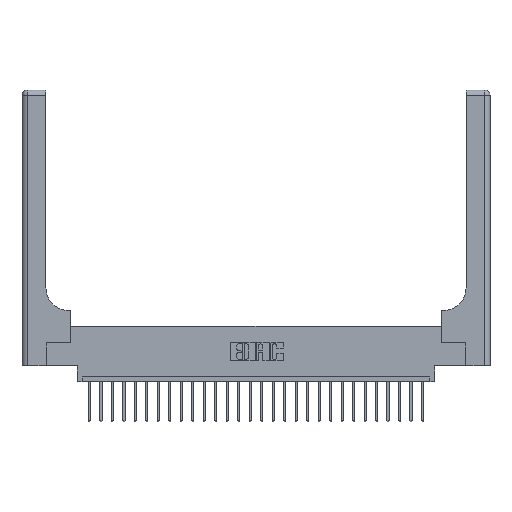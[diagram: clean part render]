
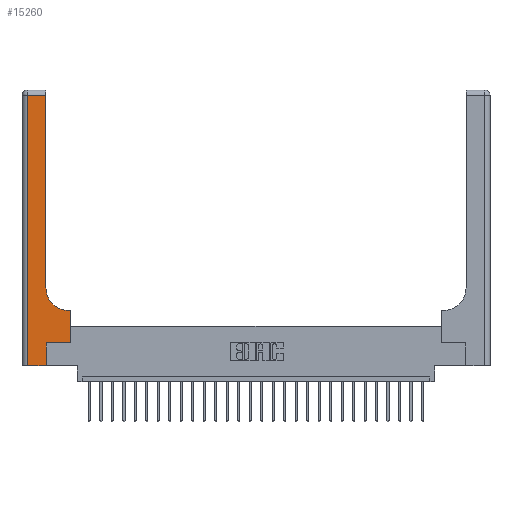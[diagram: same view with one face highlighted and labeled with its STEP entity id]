
A CAD part, top view. The second image highlights one B-rep face of the part: STEP entity #15260.
In plain terms, the highlighted planar face has unit normal (0, 0, 1).
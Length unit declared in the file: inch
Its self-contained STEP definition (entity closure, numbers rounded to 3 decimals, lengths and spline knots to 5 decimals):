
#6 = VERTEX_POINT ( 'NONE', #24282 ) ;
#152 = VECTOR ( 'NONE', #21282, 39.37008 ) ;
#178 = VECTOR ( 'NONE', #401, 39.37008 ) ;
#401 = DIRECTION ( 'NONE',  ( 0., 1., 0. ) ) ;
#1646 = EDGE_CURVE ( 'NONE', #12417, #21705, #16898, .T. ) ;
#3020 = VERTEX_POINT ( 'NONE', #6856 ) ;
#3327 = VECTOR ( 'NONE', #15377, 39.37008 ) ;
#3808 = EDGE_CURVE ( 'NONE', #14469, #10279, #16471, .T. ) ;
#3877 = ORIENTED_EDGE ( 'NONE', *, *, #6698, .T. ) ;
#3986 = EDGE_LOOP ( 'NONE', ( #5936, #6152, #3877, #6165, #24471, #15004, #22845, #21467, #20799 ) ) ;
#4319 = PLANE ( 'NONE',  #25416 ) ;
#4396 = CARTESIAN_POINT ( 'NONE',  ( 0.51, 0.6, 0.37 ) ) ;
#4500 = VERTEX_POINT ( 'NONE', #19045 ) ;
#4803 = CARTESIAN_POINT ( 'NONE',  ( 0., 0., 0.37 ) ) ;
#5450 = EDGE_CURVE ( 'NONE', #25937, #3020, #11357, .T. ) ;
#5936 = ORIENTED_EDGE ( 'NONE', *, *, #3808, .T. ) ;
#6042 = DIRECTION ( 'NONE',  ( 0., 0., -1. ) ) ;
#6152 = ORIENTED_EDGE ( 'NONE', *, *, #19553, .T. ) ;
#6165 = ORIENTED_EDGE ( 'NONE', *, *, #1646, .T. ) ;
#6204 = LINE ( 'NONE', #7906, #25130 ) ;
#6209 = CARTESIAN_POINT ( 'NONE',  ( 0.26, 3., 0.37 ) ) ;
#6305 = EDGE_CURVE ( 'NONE', #18394, #14469, #23410, .T. ) ;
#6698 = EDGE_CURVE ( 'NONE', #6, #12417, #6204, .T. ) ;
#6782 = VECTOR ( 'NONE', #19073, 39.37008 ) ;
#6834 = CARTESIAN_POINT ( 'NONE',  ( 0.265, 0., 0.37 ) ) ;
#6856 = CARTESIAN_POINT ( 'NONE',  ( 0.528, 0.25, 0.37 ) ) ;
#7074 = EDGE_CURVE ( 'NONE', #3020, #4500, #9326, .T. ) ;
#7271 = DIRECTION ( 'NONE',  ( 1., 0., 0. ) ) ;
#7906 = CARTESIAN_POINT ( 'NONE',  ( 0.06, 3., 0.37 ) ) ;
#8956 = LINE ( 'NONE', #16983, #6782 ) ;
#9162 = DIRECTION ( 'NONE',  ( 0., 0., -1. ) ) ;
#9287 = CARTESIAN_POINT ( 'NONE',  ( 0.51, 0.85, 0.37 ) ) ;
#9326 = LINE ( 'NONE', #14016, #3327 ) ;
#10279 = VERTEX_POINT ( 'NONE', #18999 ) ;
#11066 = CARTESIAN_POINT ( 'NONE',  ( 0.26, 0.6, 0.37 ) ) ;
#11341 = VECTOR ( 'NONE', #7271, 39.37008 ) ;
#11357 = LINE ( 'NONE', #20954, #11341 ) ;
#11573 = LINE ( 'NONE', #11066, #17942 ) ;
#12201 = CARTESIAN_POINT ( 'NONE',  ( 0.26, 0.85, 0.37 ) ) ;
#12417 = VERTEX_POINT ( 'NONE', #12977 ) ;
#12820 = DIRECTION ( 'NONE',  ( 1., 0., 0. ) ) ;
#12935 = AXIS2_PLACEMENT_3D ( 'NONE', #9287, #9162, #19528 ) ;
#12977 = CARTESIAN_POINT ( 'NONE',  ( 0.06, 0., 0.37 ) ) ;
#14016 = CARTESIAN_POINT ( 'NONE',  ( 0.528, 0.25, 0.37 ) ) ;
#14325 = FACE_OUTER_BOUND ( 'NONE', #3986, .T. ) ;
#14469 = VERTEX_POINT ( 'NONE', #12201 ) ;
#15004 = ORIENTED_EDGE ( 'NONE', *, *, #5450, .T. ) ;
#15260 = ADVANCED_FACE ( 'NONE', ( #14325 ), #4319, .F. ) ;
#15377 = DIRECTION ( 'NONE',  ( 0., 1., 0. ) ) ;
#15930 = DIRECTION ( 'NONE',  ( 0., -1., 0. ) ) ;
#16024 = CARTESIAN_POINT ( 'NONE',  ( 0., 3., 0.37 ) ) ;
#16471 = LINE ( 'NONE', #6209, #178 ) ;
#16898 = LINE ( 'NONE', #4803, #24745 ) ;
#16983 = CARTESIAN_POINT ( 'NONE',  ( 0., 2.94, 0.37 ) ) ;
#17853 = EDGE_CURVE ( 'NONE', #4500, #18394, #11573, .T. ) ;
#17942 = VECTOR ( 'NONE', #19077, 39.37008 ) ;
#18394 = VERTEX_POINT ( 'NONE', #4396 ) ;
#18999 = CARTESIAN_POINT ( 'NONE',  ( 0.26, 2.94, 0.37 ) ) ;
#19045 = CARTESIAN_POINT ( 'NONE',  ( 0.528, 0.6, 0.37 ) ) ;
#19049 = LINE ( 'NONE', #6834, #152 ) ;
#19073 = DIRECTION ( 'NONE',  ( -1., 0., 0. ) ) ;
#19077 = DIRECTION ( 'NONE',  ( -1., 0., 0. ) ) ;
#19160 = DIRECTION ( 'NONE',  ( -1., 0., 0. ) ) ;
#19528 = DIRECTION ( 'NONE',  ( 1., 0., 0. ) ) ;
#19553 = EDGE_CURVE ( 'NONE', #10279, #6, #8956, .T. ) ;
#19908 = CARTESIAN_POINT ( 'NONE',  ( 0.265, 0., 0.37 ) ) ;
#20799 = ORIENTED_EDGE ( 'NONE', *, *, #6305, .T. ) ;
#20947 = CARTESIAN_POINT ( 'NONE',  ( 0.265, 0.25, 0.37 ) ) ;
#20954 = CARTESIAN_POINT ( 'NONE',  ( 0.265, 0.25, 0.37 ) ) ;
#21282 = DIRECTION ( 'NONE',  ( 0., 1., 0. ) ) ;
#21467 = ORIENTED_EDGE ( 'NONE', *, *, #17853, .T. ) ;
#21705 = VERTEX_POINT ( 'NONE', #19908 ) ;
#22360 = EDGE_CURVE ( 'NONE', #21705, #25937, #19049, .T. ) ;
#22845 = ORIENTED_EDGE ( 'NONE', *, *, #7074, .T. ) ;
#23410 = CIRCLE ( 'NONE', #12935, 0.25 ) ;
#24282 = CARTESIAN_POINT ( 'NONE',  ( 0.06, 2.94, 0.37 ) ) ;
#24471 = ORIENTED_EDGE ( 'NONE', *, *, #22360, .T. ) ;
#24745 = VECTOR ( 'NONE', #12820, 39.37008 ) ;
#25130 = VECTOR ( 'NONE', #15930, 39.37008 ) ;
#25416 = AXIS2_PLACEMENT_3D ( 'NONE', #16024, #6042, #19160 ) ;
#25937 = VERTEX_POINT ( 'NONE', #20947 ) ;
